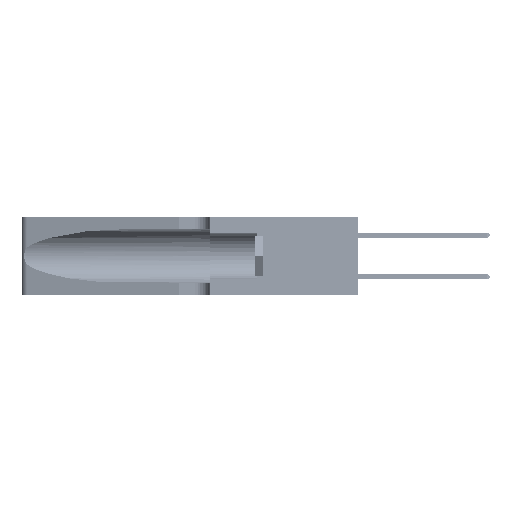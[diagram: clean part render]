
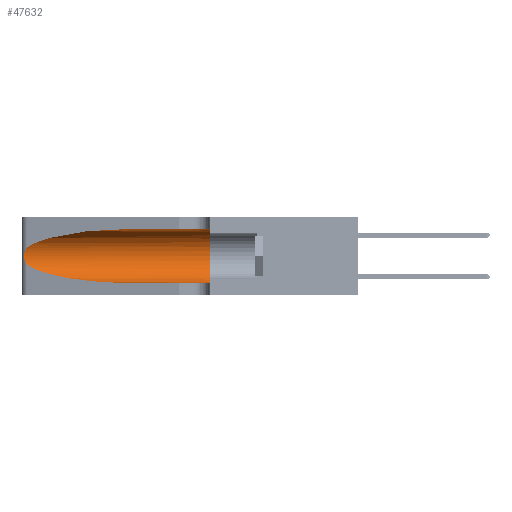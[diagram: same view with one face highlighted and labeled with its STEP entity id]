
A CAD part, left-side view. The second image highlights one B-rep face of the part: STEP entity #47632.
In plain terms, the highlighted cylindrical face has radius 3.308 mm (diameter 6.617 mm), a partial arc.
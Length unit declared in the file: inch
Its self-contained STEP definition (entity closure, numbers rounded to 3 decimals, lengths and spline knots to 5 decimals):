
#254 = DIRECTION ( 'NONE',  ( 0., 0., -1. ) ) ;
#1293 = VECTOR ( 'NONE', #49714, 39.37008 ) ;
#1303 = CARTESIAN_POINT ( 'NONE',  ( 0.26018, 1.23835, 0.19895 ) ) ;
#1624 = VERTEX_POINT ( 'NONE', #36690 ) ;
#1978 = CARTESIAN_POINT ( 'NONE',  ( 0.25639, 1.23184, 0.21858 ) ) ;
#3547 = CARTESIAN_POINT ( 'NONE',  ( 0.18966, 0.96281, 0.05475 ) ) ;
#3565 = VERTEX_POINT ( 'NONE', #21636 ) ;
#4125 = CARTESIAN_POINT ( 'NONE',  ( 0.1305, 0.72297, 0.05475 ) ) ;
#5192 = CARTESIAN_POINT ( 'NONE',  ( 0.26075, 1.23896, 0.19203 ) ) ;
#5298 = CARTESIAN_POINT ( 'NONE',  ( 0.25487, 1.22718, 0.14631 ) ) ;
#6029 = CARTESIAN_POINT ( 'NONE',  ( 0.25487, 1.22718, 0.14631 ) ) ;
#7446 = ORIENTED_EDGE ( 'NONE', *, *, #43579, .F. ) ;
#7920 =( BOUNDED_CURVE ( )  B_SPLINE_CURVE ( 3, ( #8854, #20544, #41377, #18398 ),
 .UNSPECIFIED., .F., .F. ) 
 B_SPLINE_CURVE_WITH_KNOTS ( ( 4, 4 ),
 ( 1.5708, 2.84003 ),
 .UNSPECIFIED. ) 
 CURVE ( )  GEOMETRIC_REPRESENTATION_ITEM ( )  RATIONAL_B_SPLINE_CURVE ( ( 1., 0.87, 0.87, 1. ) ) 
 REPRESENTATION_ITEM ( '' )  );
#8854 = CARTESIAN_POINT ( 'NONE',  ( 0.1305, 0.72297, 0.31525 ) ) ;
#9090 = CARTESIAN_POINT ( 'NONE',  ( 0.26075, 1.23896, 0.178 ) ) ;
#9255 = CARTESIAN_POINT ( 'NONE',  ( 0.25639, 1.23186, 0.15144 ) ) ;
#9433 = CARTESIAN_POINT ( 'NONE',  ( 0.25555, 1.22993, 0.14849 ) ) ;
#10346 = VERTEX_POINT ( 'NONE', #45128 ) ;
#10918 = VECTOR ( 'NONE', #13832, 39.37008 ) ;
#11371 = DIRECTION ( 'NONE',  ( 0., 1., 0. ) ) ;
#11462 = VERTEX_POINT ( 'NONE', #4125 ) ;
#11590 = EDGE_CURVE ( 'NONE', #1624, #38571, #7920, .T. ) ;
#12537 = EDGE_CURVE ( 'NONE', #11462, #3565, #29103, .T. ) ;
#12999 = CARTESIAN_POINT ( 'NONE',  ( 0.1305, 0.72297, 0.05475 ) ) ;
#13156 = CARTESIAN_POINT ( 'NONE',  ( 0.25789, 1.23486, 0.15765 ) ) ;
#13832 = DIRECTION ( 'NONE',  ( 0., -1., 0. ) ) ;
#14497 = VERTEX_POINT ( 'NONE', #6029 ) ;
#14550 = ORIENTED_EDGE ( 'NONE', *, *, #12537, .T. ) ;
#14753 = B_SPLINE_CURVE_WITH_KNOTS ( 'NONE', 3,
 ( #28603, #16867, #1978, #43920, #48153, #1303, #5192, #9090, #40136, #32507, #13156, #9255, #9433, #36557 ),
 .UNSPECIFIED., .F., .F.,
 ( 4, 2, 2, 2, 2, 2, 4 ),
 ( 0., 0.00027, 0.00053, 0.00107, 0.0016, 0.00187, 0.00214 ),
 .UNSPECIFIED. ) ;
#14925 = EDGE_CURVE ( 'NONE', #14497, #11462, #49333, .T. ) ;
#15246 = CARTESIAN_POINT ( 'NONE',  ( 0.1305, 0.35, 0.185 ) ) ;
#16867 = CARTESIAN_POINT ( 'NONE',  ( 0.25555, 1.22994, 0.2215 ) ) ;
#17687 = ORIENTED_EDGE ( 'NONE', *, *, #11590, .T. ) ;
#18398 = CARTESIAN_POINT ( 'NONE',  ( 0.25487, 1.22718, 0.22369 ) ) ;
#19023 = ORIENTED_EDGE ( 'NONE', *, *, #14925, .T. ) ;
#19603 = EDGE_LOOP ( 'NONE', ( #17687, #43808, #19023, #14550, #38342, #7446 ) ) ;
#20544 = CARTESIAN_POINT ( 'NONE',  ( 0.18966, 0.96281, 0.31525 ) ) ;
#21636 = CARTESIAN_POINT ( 'NONE',  ( 0.1305, 0.35, 0.05475 ) ) ;
#21907 = LINE ( 'NONE', #38152, #1293 ) ;
#23798 = CARTESIAN_POINT ( 'NONE',  ( 0.1305, 1.61858, 0.185 ) ) ;
#24838 = FACE_OUTER_BOUND ( 'NONE', #19603, .T. ) ;
#25173 = EDGE_CURVE ( 'NONE', #38571, #14497, #14753, .T. ) ;
#26791 = CARTESIAN_POINT ( 'NONE',  ( 0.2373, 1.15595, 0.08982 ) ) ;
#28603 = CARTESIAN_POINT ( 'NONE',  ( 0.25487, 1.22718, 0.22369 ) ) ;
#29103 = LINE ( 'NONE', #40508, #10918 ) ;
#30283 = EDGE_CURVE ( 'NONE', #10346, #3565, #46532, .T. ) ;
#31605 = DIRECTION ( 'NONE',  ( 0., -1., 0. ) ) ;
#32507 = CARTESIAN_POINT ( 'NONE',  ( 0.25856, 1.23593, 0.16098 ) ) ;
#32561 = CARTESIAN_POINT ( 'NONE',  ( 0.25487, 1.22718, 0.22369 ) ) ;
#36557 = CARTESIAN_POINT ( 'NONE',  ( 0.25487, 1.22718, 0.14631 ) ) ;
#36690 = CARTESIAN_POINT ( 'NONE',  ( 0.1305, 0.72297, 0.31525 ) ) ;
#38152 = CARTESIAN_POINT ( 'NONE',  ( 0.1305, 1.61858, 0.31525 ) ) ;
#38342 = ORIENTED_EDGE ( 'NONE', *, *, #30283, .F. ) ;
#38571 = VERTEX_POINT ( 'NONE', #32561 ) ;
#40136 = CARTESIAN_POINT ( 'NONE',  ( 0.26017, 1.23833, 0.17102 ) ) ;
#40508 = CARTESIAN_POINT ( 'NONE',  ( 0.1305, 1.61858, 0.05475 ) ) ;
#41377 = CARTESIAN_POINT ( 'NONE',  ( 0.2373, 1.15595, 0.28018 ) ) ;
#43579 = EDGE_CURVE ( 'NONE', #1624, #10346, #21907, .T. ) ;
#43808 = ORIENTED_EDGE ( 'NONE', *, *, #25173, .T. ) ;
#43920 = CARTESIAN_POINT ( 'NONE',  ( 0.25787, 1.23484, 0.2124 ) ) ;
#44306 = CYLINDRICAL_SURFACE ( 'NONE', #46667, 0.13025 ) ;
#45128 = CARTESIAN_POINT ( 'NONE',  ( 0.1305, 0.35, 0.31525 ) ) ;
#45841 = AXIS2_PLACEMENT_3D ( 'NONE', #15246, #11371, #46003 ) ;
#46003 = DIRECTION ( 'NONE',  ( 0., 0., 1. ) ) ;
#46532 = CIRCLE ( 'NONE', #45841, 0.13025 ) ;
#46667 = AXIS2_PLACEMENT_3D ( 'NONE', #23798, #31605, #254 ) ;
#47632 = ADVANCED_FACE ( 'NONE', ( #24838 ), #44306, .F. ) ;
#48153 = CARTESIAN_POINT ( 'NONE',  ( 0.25854, 1.2359, 0.20912 ) ) ;
#49333 =( BOUNDED_CURVE ( )  B_SPLINE_CURVE ( 3, ( #5298, #26791, #3547, #12999 ),
 .UNSPECIFIED., .F., .T. ) 
 B_SPLINE_CURVE_WITH_KNOTS ( ( 4, 4 ),
 ( 3.44316, 4.71239 ),
 .UNSPECIFIED. ) 
 CURVE ( )  GEOMETRIC_REPRESENTATION_ITEM ( )  RATIONAL_B_SPLINE_CURVE ( ( 1., 0.87, 0.87, 1. ) ) 
 REPRESENTATION_ITEM ( '' )  );
#49714 = DIRECTION ( 'NONE',  ( 0., -1., 0. ) ) ;
